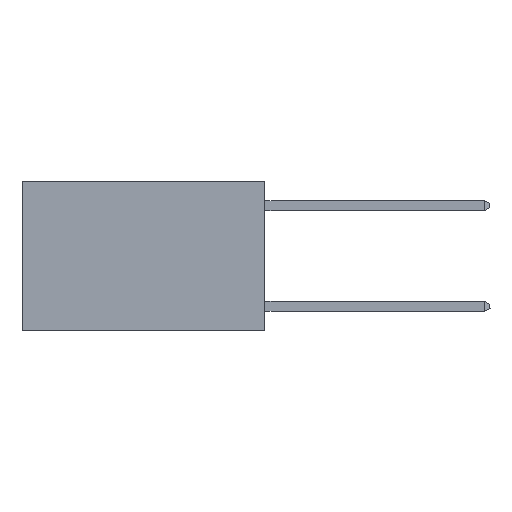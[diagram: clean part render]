
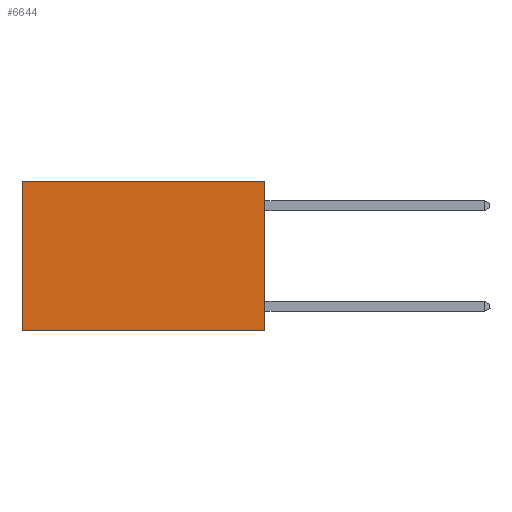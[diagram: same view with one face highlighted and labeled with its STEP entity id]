
A CAD part, left-side view. The second image highlights one B-rep face of the part: STEP entity #6644.
In plain terms, the highlighted planar face has unit normal (-1, 0, 0).
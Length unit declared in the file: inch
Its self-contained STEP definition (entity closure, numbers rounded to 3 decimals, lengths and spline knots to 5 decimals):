
#731 = EDGE_CURVE ( 'NONE', #17097, #9915, #5973, .T. ) ;
#1089 = DIRECTION ( 'NONE',  ( 0., 1., 0. ) ) ;
#1249 = VECTOR ( 'NONE', #1089, 39.37008 ) ;
#1792 = LINE ( 'NONE', #5764, #9039 ) ;
#1873 = ORIENTED_EDGE ( 'NONE', *, *, #13180, .F. ) ;
#2080 = VECTOR ( 'NONE', #10341, 39.37008 ) ;
#2198 = AXIS2_PLACEMENT_3D ( 'NONE', #6413, #15715, #7765 ) ;
#2339 = VECTOR ( 'NONE', #6439, 39.37008 ) ;
#4193 = EDGE_LOOP ( 'NONE', ( #11309, #9635, #1873, #12565 ) ) ;
#4737 = EDGE_CURVE ( 'NONE', #13921, #17097, #1792, .T. ) ;
#4970 = PLANE ( 'NONE',  #2198 ) ;
#5764 = CARTESIAN_POINT ( 'NONE',  ( 0.2625, 0., 0. ) ) ;
#5973 = LINE ( 'NONE', #6398, #2339 ) ;
#6109 = CARTESIAN_POINT ( 'NONE',  ( 0.2625, 0.6, 0. ) ) ;
#6398 = CARTESIAN_POINT ( 'NONE',  ( 0.2625, 0.6, 0. ) ) ;
#6413 = CARTESIAN_POINT ( 'NONE',  ( 0.2625, 0., 0. ) ) ;
#6439 = DIRECTION ( 'NONE',  ( 0., 0., -1. ) ) ;
#6644 = ADVANCED_FACE ( 'NONE', ( #15595 ), #4970, .F. ) ;
#7765 = DIRECTION ( 'NONE',  ( 0., 0., -1. ) ) ;
#9001 = CARTESIAN_POINT ( 'NONE',  ( 0.2625, 0., 0. ) ) ;
#9039 = VECTOR ( 'NONE', #16401, 39.37008 ) ;
#9635 = ORIENTED_EDGE ( 'NONE', *, *, #12775, .F. ) ;
#9915 = VERTEX_POINT ( 'NONE', #14048 ) ;
#10341 = DIRECTION ( 'NONE',  ( 0., 0., -1. ) ) ;
#11309 = ORIENTED_EDGE ( 'NONE', *, *, #731, .T. ) ;
#11804 = CARTESIAN_POINT ( 'NONE',  ( 0.2625, 0., 0. ) ) ;
#12565 = ORIENTED_EDGE ( 'NONE', *, *, #4737, .T. ) ;
#12747 = CARTESIAN_POINT ( 'NONE',  ( 0.2625, 0., -0.37 ) ) ;
#12775 = EDGE_CURVE ( 'NONE', #16389, #9915, #15133, .T. ) ;
#13180 = EDGE_CURVE ( 'NONE', #13921, #16389, #13708, .T. ) ;
#13708 = LINE ( 'NONE', #9001, #2080 ) ;
#13921 = VERTEX_POINT ( 'NONE', #11804 ) ;
#14048 = CARTESIAN_POINT ( 'NONE',  ( 0.2625, 0.6, -0.37 ) ) ;
#15133 = LINE ( 'NONE', #15836, #1249 ) ;
#15595 = FACE_OUTER_BOUND ( 'NONE', #4193, .T. ) ;
#15715 = DIRECTION ( 'NONE',  ( 1., 0., 0. ) ) ;
#15836 = CARTESIAN_POINT ( 'NONE',  ( 0.2625, 0., -0.37 ) ) ;
#16389 = VERTEX_POINT ( 'NONE', #12747 ) ;
#16401 = DIRECTION ( 'NONE',  ( 0., 1., 0. ) ) ;
#17097 = VERTEX_POINT ( 'NONE', #6109 ) ;
